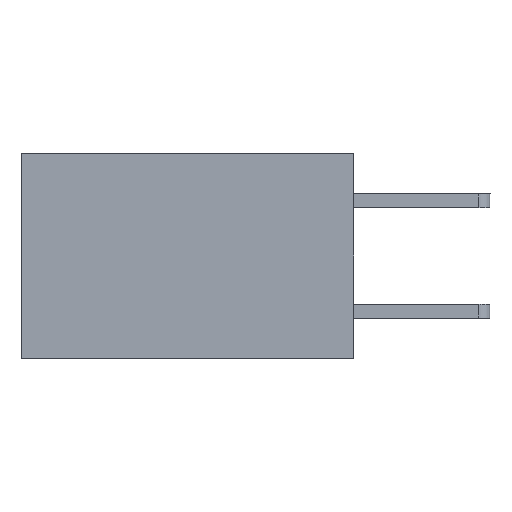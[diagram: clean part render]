
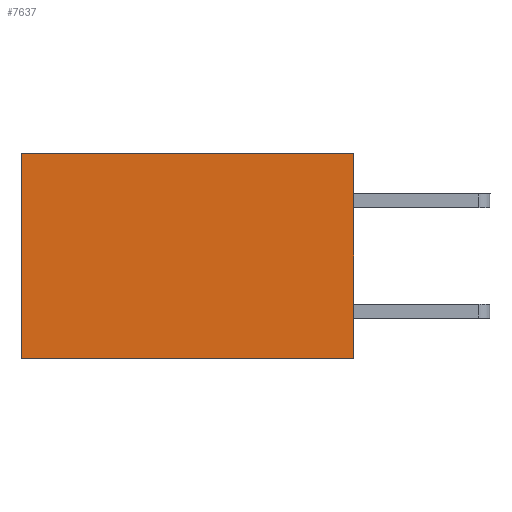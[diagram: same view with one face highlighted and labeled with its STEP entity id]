
A CAD part, left-side view. The second image highlights one B-rep face of the part: STEP entity #7637.
In plain terms, the highlighted planar face has unit normal (-1, 0, 0).
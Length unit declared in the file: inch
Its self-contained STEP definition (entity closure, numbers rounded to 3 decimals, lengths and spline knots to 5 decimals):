
#12 = DIRECTION ( 'NONE',  ( 0., 1., 0. ) ) ;
#468 = LINE ( 'NONE', #9280, #8488 ) ;
#957 = CARTESIAN_POINT ( 'NONE',  ( 0.2875, 0.6, 0. ) ) ;
#1268 = DIRECTION ( 'NONE',  ( 0., 1., 0. ) ) ;
#1356 = EDGE_LOOP ( 'NONE', ( #2466, #7341, #3577, #7301 ) ) ;
#1588 = VECTOR ( 'NONE', #12, 39.37008 ) ;
#1667 = EDGE_CURVE ( 'NONE', #1836, #5540, #468, .T. ) ;
#1836 = VERTEX_POINT ( 'NONE', #3778 ) ;
#1844 = CARTESIAN_POINT ( 'NONE',  ( 0.2875, 0., -0.37 ) ) ;
#2153 = LINE ( 'NONE', #3431, #3921 ) ;
#2246 = LINE ( 'NONE', #1844, #1588 ) ;
#2445 = AXIS2_PLACEMENT_3D ( 'NONE', #6727, #4552, #9719 ) ;
#2466 = ORIENTED_EDGE ( 'NONE', *, *, #4961, .T. ) ;
#2634 = CARTESIAN_POINT ( 'NONE',  ( 0.2875, 0., -0.37 ) ) ;
#3232 = VECTOR ( 'NONE', #6509, 39.37008 ) ;
#3250 = DIRECTION ( 'NONE',  ( 0., 0., -1. ) ) ;
#3431 = CARTESIAN_POINT ( 'NONE',  ( 0.2875, 0.6, 0. ) ) ;
#3577 = ORIENTED_EDGE ( 'NONE', *, *, #3996, .F. ) ;
#3778 = CARTESIAN_POINT ( 'NONE',  ( 0.2875, 0., 0. ) ) ;
#3810 = PLANE ( 'NONE',  #2445 ) ;
#3921 = VECTOR ( 'NONE', #3250, 39.37008 ) ;
#3996 = EDGE_CURVE ( 'NONE', #1836, #6888, #8990, .T. ) ;
#4331 = FACE_OUTER_BOUND ( 'NONE', #1356, .T. ) ;
#4552 = DIRECTION ( 'NONE',  ( 1., 0., 0. ) ) ;
#4961 = EDGE_CURVE ( 'NONE', #5540, #9252, #2153, .T. ) ;
#5540 = VERTEX_POINT ( 'NONE', #957 ) ;
#5763 = CARTESIAN_POINT ( 'NONE',  ( 0.2875, 0.6, -0.37 ) ) ;
#6254 = EDGE_CURVE ( 'NONE', #6888, #9252, #2246, .T. ) ;
#6509 = DIRECTION ( 'NONE',  ( 0., 0., -1. ) ) ;
#6546 = CARTESIAN_POINT ( 'NONE',  ( 0.2875, 0., 0. ) ) ;
#6727 = CARTESIAN_POINT ( 'NONE',  ( 0.2875, 0., 0. ) ) ;
#6888 = VERTEX_POINT ( 'NONE', #2634 ) ;
#7301 = ORIENTED_EDGE ( 'NONE', *, *, #1667, .T. ) ;
#7341 = ORIENTED_EDGE ( 'NONE', *, *, #6254, .F. ) ;
#7637 = ADVANCED_FACE ( 'NONE', ( #4331 ), #3810, .F. ) ;
#8488 = VECTOR ( 'NONE', #1268, 39.37008 ) ;
#8990 = LINE ( 'NONE', #6546, #3232 ) ;
#9252 = VERTEX_POINT ( 'NONE', #5763 ) ;
#9280 = CARTESIAN_POINT ( 'NONE',  ( 0.2875, 0., 0. ) ) ;
#9719 = DIRECTION ( 'NONE',  ( 0., 0., -1. ) ) ;
